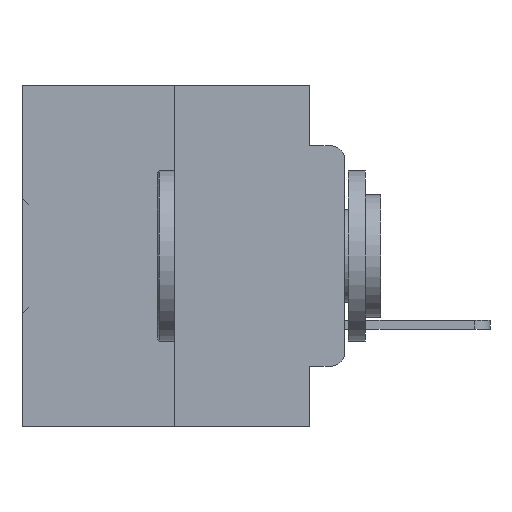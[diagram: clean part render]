
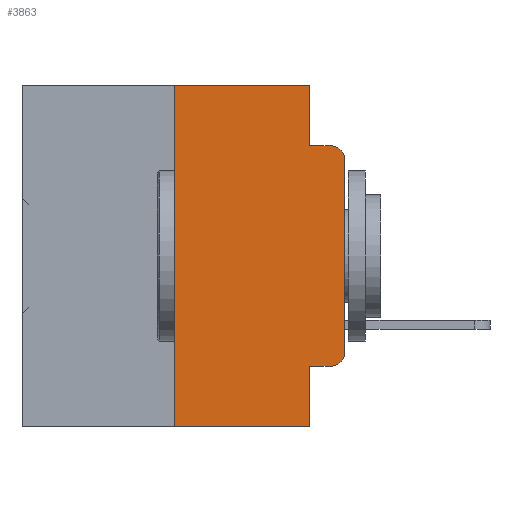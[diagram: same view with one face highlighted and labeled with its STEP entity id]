
A CAD part, left-side view. The second image highlights one B-rep face of the part: STEP entity #3863.
In plain terms, the highlighted planar face has unit normal (-1, 0, 0).
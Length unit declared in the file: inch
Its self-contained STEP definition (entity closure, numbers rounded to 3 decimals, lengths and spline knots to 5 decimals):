
#605 = DIRECTION ( 'NONE',  ( 0., -1., 0. ) ) ;
#989 = VERTEX_POINT ( 'NONE', #6657 ) ;
#1082 = DIRECTION ( 'NONE',  ( 0., 0., 1. ) ) ;
#1784 = VECTOR ( 'NONE', #29653, 39.37008 ) ;
#1857 = VERTEX_POINT ( 'NONE', #12429 ) ;
#2241 = VERTEX_POINT ( 'NONE', #29372 ) ;
#2603 = CARTESIAN_POINT ( 'NONE',  ( 0., 0.051, -0.4115 ) ) ;
#2665 = ORIENTED_EDGE ( 'NONE', *, *, #23293, .T. ) ;
#3214 = VERTEX_POINT ( 'NONE', #14665 ) ;
#3863 = ADVANCED_FACE ( 'NONE', ( #21601 ), #20579, .F. ) ;
#3924 = DIRECTION ( 'NONE',  ( 0., -1., 0. ) ) ;
#4111 = VECTOR ( 'NONE', #5676, 39.37008 ) ;
#4405 = ORIENTED_EDGE ( 'NONE', *, *, #16408, .T. ) ;
#4702 = DIRECTION ( 'NONE',  ( 0., 0., 1. ) ) ;
#5458 = CARTESIAN_POINT ( 'NONE',  ( 0., 0.02, -0.0885 ) ) ;
#5651 = AXIS2_PLACEMENT_3D ( 'NONE', #14118, #33246, #16983 ) ;
#5676 = DIRECTION ( 'NONE',  ( 0., -1., 0. ) ) ;
#5934 = CARTESIAN_POINT ( 'NONE',  ( 0., 0.25, 0. ) ) ;
#6585 = CARTESIAN_POINT ( 'NONE',  ( 0., 0.051, 0. ) ) ;
#6657 = CARTESIAN_POINT ( 'NONE',  ( 0., 0.051, 0. ) ) ;
#6888 = VECTOR ( 'NONE', #1082, 39.37008 ) ;
#7279 = CARTESIAN_POINT ( 'NONE',  ( 0., 0.25, 0. ) ) ;
#7489 = ORIENTED_EDGE ( 'NONE', *, *, #26223, .F. ) ;
#7663 = ORIENTED_EDGE ( 'NONE', *, *, #30047, .F. ) ;
#7667 = EDGE_CURVE ( 'NONE', #22727, #1857, #24076, .T. ) ;
#7954 = CARTESIAN_POINT ( 'NONE',  ( 0., 0., -0.1085 ) ) ;
#8618 = CARTESIAN_POINT ( 'NONE',  ( 0., 0.051, -0.0885 ) ) ;
#9545 = VECTOR ( 'NONE', #4702, 39.37008 ) ;
#9771 = LINE ( 'NONE', #7279, #6888 ) ;
#9955 = LINE ( 'NONE', #25551, #1784 ) ;
#10348 = LINE ( 'NONE', #21644, #32607 ) ;
#10945 = AXIS2_PLACEMENT_3D ( 'NONE', #14209, #33325, #17072 ) ;
#11039 = VERTEX_POINT ( 'NONE', #33602 ) ;
#11462 = ORIENTED_EDGE ( 'NONE', *, *, #31157, .T. ) ;
#11580 = ORIENTED_EDGE ( 'NONE', *, *, #7667, .T. ) ;
#11777 = DIRECTION ( 'NONE',  ( 0., -1., 0. ) ) ;
#12429 = CARTESIAN_POINT ( 'NONE',  ( 0., 0., -0.3915 ) ) ;
#12610 = EDGE_CURVE ( 'NONE', #3214, #24496, #9771, .T. ) ;
#14118 = CARTESIAN_POINT ( 'NONE',  ( 0., 0.02, -0.1085 ) ) ;
#14209 = CARTESIAN_POINT ( 'NONE',  ( 0., 0.02, -0.3915 ) ) ;
#14665 = CARTESIAN_POINT ( 'NONE',  ( 0., 0.25, -0.5 ) ) ;
#15246 = LINE ( 'NONE', #15873, #29034 ) ;
#15772 = DIRECTION ( 'NONE',  ( 0., 0., -1. ) ) ;
#15873 = CARTESIAN_POINT ( 'NONE',  ( 0., 0.473, 0. ) ) ;
#16408 = EDGE_CURVE ( 'NONE', #3214, #26362, #10348, .T. ) ;
#16983 = DIRECTION ( 'NONE',  ( 0., 0., -1. ) ) ;
#17008 = AXIS2_PLACEMENT_3D ( 'NONE', #30388, #20657, #20662 ) ;
#17072 = DIRECTION ( 'NONE',  ( 0., 0., -1. ) ) ;
#17152 = CARTESIAN_POINT ( 'NONE',  ( 0., 0.02, -0.4115 ) ) ;
#18149 = CARTESIAN_POINT ( 'NONE',  ( 0., 0.051, -0.5 ) ) ;
#18675 = ORIENTED_EDGE ( 'NONE', *, *, #29727, .F. ) ;
#18881 = ORIENTED_EDGE ( 'NONE', *, *, #31616, .T. ) ;
#19418 = ORIENTED_EDGE ( 'NONE', *, *, #12610, .F. ) ;
#19958 = LINE ( 'NONE', #2603, #4111 ) ;
#20378 = ORIENTED_EDGE ( 'NONE', *, *, #24649, .F. ) ;
#20579 = PLANE ( 'NONE',  #17008 ) ;
#20657 = DIRECTION ( 'NONE',  ( 1., 0., 0. ) ) ;
#20662 = DIRECTION ( 'NONE',  ( 0., 0., -1. ) ) ;
#21601 = FACE_OUTER_BOUND ( 'NONE', #26714, .T. ) ;
#21644 = CARTESIAN_POINT ( 'NONE',  ( 0., 0.473, -0.5 ) ) ;
#22449 = CARTESIAN_POINT ( 'NONE',  ( 0., 0., 0. ) ) ;
#22727 = VERTEX_POINT ( 'NONE', #17152 ) ;
#23293 = EDGE_CURVE ( 'NONE', #1857, #30994, #30286, .T. ) ;
#23438 = VECTOR ( 'NONE', #15772, 39.37008 ) ;
#24076 = CIRCLE ( 'NONE', #10945, 0.02 ) ;
#24298 = LINE ( 'NONE', #6585, #23438 ) ;
#24496 = VERTEX_POINT ( 'NONE', #5934 ) ;
#24649 = EDGE_CURVE ( 'NONE', #989, #2241, #24298, .T. ) ;
#25551 = CARTESIAN_POINT ( 'NONE',  ( 0., 0.051, 0. ) ) ;
#26223 = EDGE_CURVE ( 'NONE', #2241, #32408, #27136, .T. ) ;
#26362 = VERTEX_POINT ( 'NONE', #18149 ) ;
#26714 = EDGE_LOOP ( 'NONE', ( #2665, #18881, #7489, #20378, #18675, #19418, #4405, #7663, #11462, #11580 ) ) ;
#27136 = LINE ( 'NONE', #8618, #33338 ) ;
#28123 = CIRCLE ( 'NONE', #5651, 0.02 ) ;
#29034 = VECTOR ( 'NONE', #605, 39.37008 ) ;
#29372 = CARTESIAN_POINT ( 'NONE',  ( 0., 0.051, -0.0885 ) ) ;
#29653 = DIRECTION ( 'NONE',  ( 0., 0., -1. ) ) ;
#29727 = EDGE_CURVE ( 'NONE', #24496, #989, #15246, .T. ) ;
#30047 = EDGE_CURVE ( 'NONE', #11039, #26362, #9955, .T. ) ;
#30286 = LINE ( 'NONE', #22449, #9545 ) ;
#30388 = CARTESIAN_POINT ( 'NONE',  ( 0., 0.473, 0. ) ) ;
#30994 = VERTEX_POINT ( 'NONE', #7954 ) ;
#31157 = EDGE_CURVE ( 'NONE', #11039, #22727, #19958, .T. ) ;
#31616 = EDGE_CURVE ( 'NONE', #30994, #32408, #28123, .T. ) ;
#32408 = VERTEX_POINT ( 'NONE', #5458 ) ;
#32607 = VECTOR ( 'NONE', #3924, 39.37008 ) ;
#33246 = DIRECTION ( 'NONE',  ( -1., 0., 0. ) ) ;
#33325 = DIRECTION ( 'NONE',  ( -1., 0., 0. ) ) ;
#33338 = VECTOR ( 'NONE', #11777, 39.37008 ) ;
#33602 = CARTESIAN_POINT ( 'NONE',  ( 0., 0.051, -0.4115 ) ) ;
